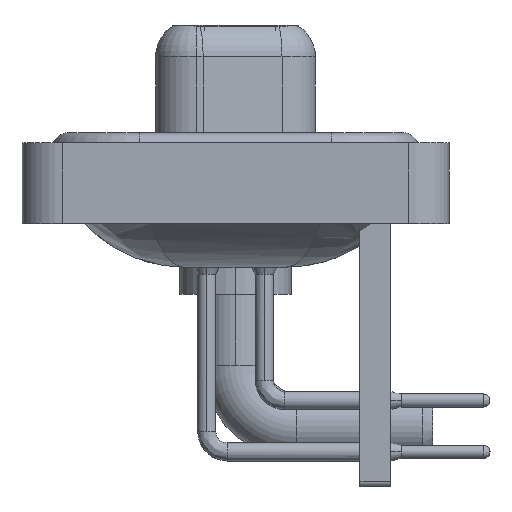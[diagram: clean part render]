
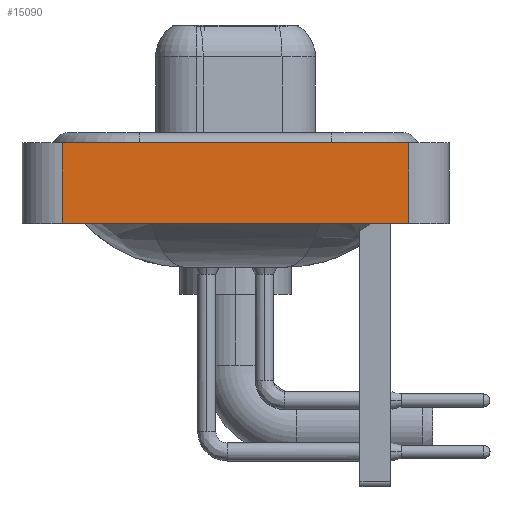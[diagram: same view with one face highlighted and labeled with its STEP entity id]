
A CAD part, left-side view. The second image highlights one B-rep face of the part: STEP entity #15090.
In plain terms, the highlighted planar face has unit normal (-1, 0, 0).
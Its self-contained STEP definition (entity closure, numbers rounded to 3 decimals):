
#760 = DIRECTION ( 'NONE',  ( 0., 0., 1. ) ) ;
#937 = LINE ( 'NONE', #26418, #17161 ) ;
#1306 = VERTEX_POINT ( 'NONE', #21404 ) ;
#2418 = CARTESIAN_POINT ( 'NONE',  ( -7.35, -8.55, 0.4 ) ) ;
#2548 = ORIENTED_EDGE ( 'NONE', *, *, #16458, .T. ) ;
#2995 = VERTEX_POINT ( 'NONE', #2418 ) ;
#3758 = DIRECTION ( 'NONE',  ( 0., 0., 1. ) ) ;
#5180 = EDGE_CURVE ( 'NONE', #1306, #11031, #25698, .T. ) ;
#7044 = CARTESIAN_POINT ( 'NONE',  ( -7.35, 8.55, 0.4 ) ) ;
#8169 = EDGE_CURVE ( 'NONE', #1306, #14703, #937, .T. ) ;
#8728 = LINE ( 'NONE', #19506, #9741 ) ;
#8846 = AXIS2_PLACEMENT_3D ( 'NONE', #26769, #18493, #3758 ) ;
#9370 = ORIENTED_EDGE ( 'NONE', *, *, #18516, .F. ) ;
#9741 = VECTOR ( 'NONE', #12593, 1000. ) ;
#11031 = VERTEX_POINT ( 'NONE', #7044 ) ;
#12038 = ORIENTED_EDGE ( 'NONE', *, *, #5180, .F. ) ;
#12187 = EDGE_LOOP ( 'NONE', ( #2548, #9370, #12038, #26404 ) ) ;
#12593 = DIRECTION ( 'NONE',  ( 0., 0., 1. ) ) ;
#12662 = DIRECTION ( 'NONE',  ( 0., -1., 0. ) ) ;
#13890 = DIRECTION ( 'NONE',  ( 0., -1., 0. ) ) ;
#14703 = VERTEX_POINT ( 'NONE', #27072 ) ;
#15090 = ADVANCED_FACE ( 'NONE', ( #16308 ), #24857, .T. ) ;
#16149 = VECTOR ( 'NONE', #12662, 1000. ) ;
#16308 = FACE_OUTER_BOUND ( 'NONE', #12187, .T. ) ;
#16458 = EDGE_CURVE ( 'NONE', #14703, #2995, #8728, .T. ) ;
#17161 = VECTOR ( 'NONE', #13890, 1000. ) ;
#18493 = DIRECTION ( 'NONE',  ( -1., 0., 0. ) ) ;
#18516 = EDGE_CURVE ( 'NONE', #11031, #2995, #19288, .T. ) ;
#19288 = LINE ( 'NONE', #23593, #16149 ) ;
#19506 = CARTESIAN_POINT ( 'NONE',  ( -7.35, -8.55, -3.6 ) ) ;
#19772 = CARTESIAN_POINT ( 'NONE',  ( -7.35, 8.55, -3.6 ) ) ;
#21404 = CARTESIAN_POINT ( 'NONE',  ( -7.35, 8.55, -3.6 ) ) ;
#22273 = VECTOR ( 'NONE', #760, 1000. ) ;
#23593 = CARTESIAN_POINT ( 'NONE',  ( -7.35, -8.55, 0.4 ) ) ;
#24857 = PLANE ( 'NONE',  #8846 ) ;
#25698 = LINE ( 'NONE', #19772, #22273 ) ;
#26404 = ORIENTED_EDGE ( 'NONE', *, *, #8169, .T. ) ;
#26418 = CARTESIAN_POINT ( 'NONE',  ( -7.35, -8.55, -3.6 ) ) ;
#26769 = CARTESIAN_POINT ( 'NONE',  ( -7.35, -8.55, -3.6 ) ) ;
#27072 = CARTESIAN_POINT ( 'NONE',  ( -7.35, -8.55, -3.6 ) ) ;
